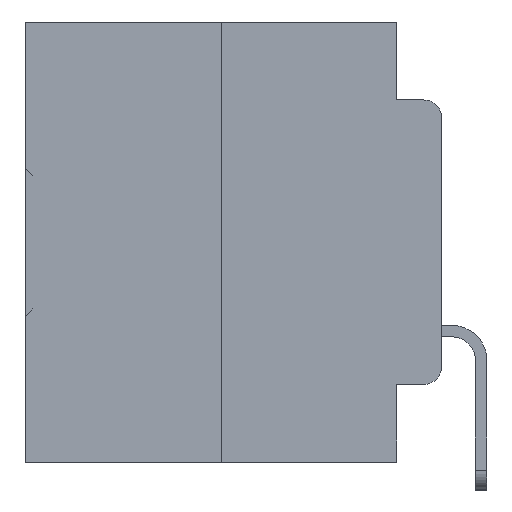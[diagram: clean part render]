
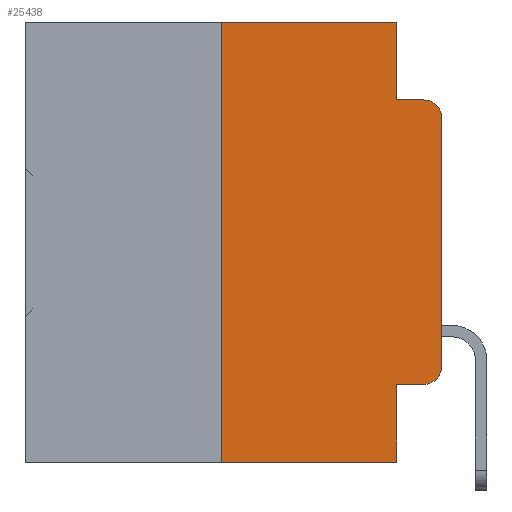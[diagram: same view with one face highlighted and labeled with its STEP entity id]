
A CAD part, left-side view. The second image highlights one B-rep face of the part: STEP entity #25438.
In plain terms, the highlighted planar face has unit normal (-1, 0, 0).
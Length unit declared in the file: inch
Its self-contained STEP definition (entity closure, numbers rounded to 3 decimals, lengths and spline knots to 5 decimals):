
#85 = CARTESIAN_POINT ( 'NONE',  ( 0., 0.051, -0.0885 ) ) ;
#91 = VERTEX_POINT ( 'NONE', #29461 ) ;
#427 = EDGE_LOOP ( 'NONE', ( #7396, #30234, #18084, #11206, #16283, #25548, #11239, #23396, #16782, #21205 ) ) ;
#664 = AXIS2_PLACEMENT_3D ( 'NONE', #36253, #22533, #5019 ) ;
#983 = LINE ( 'NONE', #20219, #8195 ) ;
#2115 = DIRECTION ( 'NONE',  ( 0., 0., -1. ) ) ;
#2241 = EDGE_CURVE ( 'NONE', #5096, #91, #11582, .T. ) ;
#2606 = CARTESIAN_POINT ( 'NONE',  ( 0., 0.25, 0. ) ) ;
#2645 = VECTOR ( 'NONE', #34446, 39.37008 ) ;
#3554 = CARTESIAN_POINT ( 'NONE',  ( 0., 0.02, -0.3915 ) ) ;
#3964 = VERTEX_POINT ( 'NONE', #14531 ) ;
#4713 = VERTEX_POINT ( 'NONE', #20827 ) ;
#5019 = DIRECTION ( 'NONE',  ( 0., 0., -1. ) ) ;
#5096 = VERTEX_POINT ( 'NONE', #13913 ) ;
#5925 = CARTESIAN_POINT ( 'NONE',  ( 0., 0.473, -0.5 ) ) ;
#6607 = DIRECTION ( 'NONE',  ( 0., 0., -1. ) ) ;
#7396 = ORIENTED_EDGE ( 'NONE', *, *, #7858, .T. ) ;
#7503 = EDGE_CURVE ( 'NONE', #15912, #3964, #19468, .T. ) ;
#7858 = EDGE_CURVE ( 'NONE', #91, #36881, #17068, .T. ) ;
#8195 = VECTOR ( 'NONE', #36746, 39.37008 ) ;
#8409 = CIRCLE ( 'NONE', #25326, 0.02 ) ;
#9127 = AXIS2_PLACEMENT_3D ( 'NONE', #3554, #24020, #6607 ) ;
#9540 = EDGE_CURVE ( 'NONE', #15912, #5096, #16025, .T. ) ;
#10411 = VECTOR ( 'NONE', #14740, 39.37008 ) ;
#10732 = LINE ( 'NONE', #5925, #2645 ) ;
#10941 = PLANE ( 'NONE',  #664 ) ;
#10994 = EDGE_CURVE ( 'NONE', #27776, #14286, #27114, .T. ) ;
#11180 = CARTESIAN_POINT ( 'NONE',  ( 0., 0., -0.1085 ) ) ;
#11206 = ORIENTED_EDGE ( 'NONE', *, *, #17180, .F. ) ;
#11239 = ORIENTED_EDGE ( 'NONE', *, *, #22356, .T. ) ;
#11582 = CIRCLE ( 'NONE', #9127, 0.02 ) ;
#11720 = VECTOR ( 'NONE', #2115, 39.37008 ) ;
#13692 = CARTESIAN_POINT ( 'NONE',  ( 0., 0.051, -0.0885 ) ) ;
#13913 = CARTESIAN_POINT ( 'NONE',  ( 0., 0.02, -0.4115 ) ) ;
#14286 = VERTEX_POINT ( 'NONE', #17672 ) ;
#14531 = CARTESIAN_POINT ( 'NONE',  ( 0., 0.051, -0.5 ) ) ;
#14740 = DIRECTION ( 'NONE',  ( 0., 0., 1. ) ) ;
#14763 = DIRECTION ( 'NONE',  ( 0., -1., 0. ) ) ;
#15865 = DIRECTION ( 'NONE',  ( -1., 0., 0. ) ) ;
#15912 = VERTEX_POINT ( 'NONE', #23491 ) ;
#16025 = LINE ( 'NONE', #19406, #31182 ) ;
#16283 = ORIENTED_EDGE ( 'NONE', *, *, #10994, .F. ) ;
#16681 = CARTESIAN_POINT ( 'NONE',  ( 0., 0.25, -0.5 ) ) ;
#16782 = ORIENTED_EDGE ( 'NONE', *, *, #9540, .T. ) ;
#16838 = VECTOR ( 'NONE', #27915, 39.37008 ) ;
#17068 = LINE ( 'NONE', #27326, #29289 ) ;
#17088 = CARTESIAN_POINT ( 'NONE',  ( 0., 0.051, 0. ) ) ;
#17180 = EDGE_CURVE ( 'NONE', #14286, #35559, #983, .T. ) ;
#17672 = CARTESIAN_POINT ( 'NONE',  ( 0., 0.051, 0. ) ) ;
#18084 = ORIENTED_EDGE ( 'NONE', *, *, #20953, .F. ) ;
#18230 = LINE ( 'NONE', #2606, #10411 ) ;
#19406 = CARTESIAN_POINT ( 'NONE',  ( 0., 0.051, -0.4115 ) ) ;
#19468 = LINE ( 'NONE', #17088, #11720 ) ;
#19719 = VECTOR ( 'NONE', #14763, 39.37008 ) ;
#20219 = CARTESIAN_POINT ( 'NONE',  ( 0., 0.051, 0. ) ) ;
#20261 = FACE_OUTER_BOUND ( 'NONE', #427, .T. ) ;
#20827 = CARTESIAN_POINT ( 'NONE',  ( 0., 0.02, -0.0885 ) ) ;
#20953 = EDGE_CURVE ( 'NONE', #35559, #4713, #24294, .T. ) ;
#21205 = ORIENTED_EDGE ( 'NONE', *, *, #2241, .T. ) ;
#21719 = DIRECTION ( 'NONE',  ( 0., 0., 1. ) ) ;
#22356 = EDGE_CURVE ( 'NONE', #35901, #3964, #10732, .T. ) ;
#22533 = DIRECTION ( 'NONE',  ( 1., 0., 0. ) ) ;
#23396 = ORIENTED_EDGE ( 'NONE', *, *, #7503, .F. ) ;
#23491 = CARTESIAN_POINT ( 'NONE',  ( 0., 0.051, -0.4115 ) ) ;
#24020 = DIRECTION ( 'NONE',  ( -1., 0., 0. ) ) ;
#24294 = LINE ( 'NONE', #13692, #16838 ) ;
#25326 = AXIS2_PLACEMENT_3D ( 'NONE', #32567, #15865, #35339 ) ;
#25438 = ADVANCED_FACE ( 'NONE', ( #20261 ), #10941, .F. ) ;
#25548 = ORIENTED_EDGE ( 'NONE', *, *, #34866, .F. ) ;
#26669 = EDGE_CURVE ( 'NONE', #36881, #4713, #8409, .T. ) ;
#27114 = LINE ( 'NONE', #37153, #19719 ) ;
#27326 = CARTESIAN_POINT ( 'NONE',  ( 0., 0., 0. ) ) ;
#27776 = VERTEX_POINT ( 'NONE', #35752 ) ;
#27915 = DIRECTION ( 'NONE',  ( 0., -1., 0. ) ) ;
#29289 = VECTOR ( 'NONE', #21719, 39.37008 ) ;
#29461 = CARTESIAN_POINT ( 'NONE',  ( 0., 0., -0.3915 ) ) ;
#30234 = ORIENTED_EDGE ( 'NONE', *, *, #26669, .T. ) ;
#31182 = VECTOR ( 'NONE', #33165, 39.37008 ) ;
#32567 = CARTESIAN_POINT ( 'NONE',  ( 0., 0.02, -0.1085 ) ) ;
#33165 = DIRECTION ( 'NONE',  ( 0., -1., 0. ) ) ;
#34446 = DIRECTION ( 'NONE',  ( 0., -1., 0. ) ) ;
#34866 = EDGE_CURVE ( 'NONE', #35901, #27776, #18230, .T. ) ;
#35339 = DIRECTION ( 'NONE',  ( 0., 0., -1. ) ) ;
#35559 = VERTEX_POINT ( 'NONE', #85 ) ;
#35752 = CARTESIAN_POINT ( 'NONE',  ( 0., 0.25, 0. ) ) ;
#35901 = VERTEX_POINT ( 'NONE', #16681 ) ;
#36253 = CARTESIAN_POINT ( 'NONE',  ( 0., 0.473, 0. ) ) ;
#36746 = DIRECTION ( 'NONE',  ( 0., 0., -1. ) ) ;
#36881 = VERTEX_POINT ( 'NONE', #11180 ) ;
#37153 = CARTESIAN_POINT ( 'NONE',  ( 0., 0.473, 0. ) ) ;
